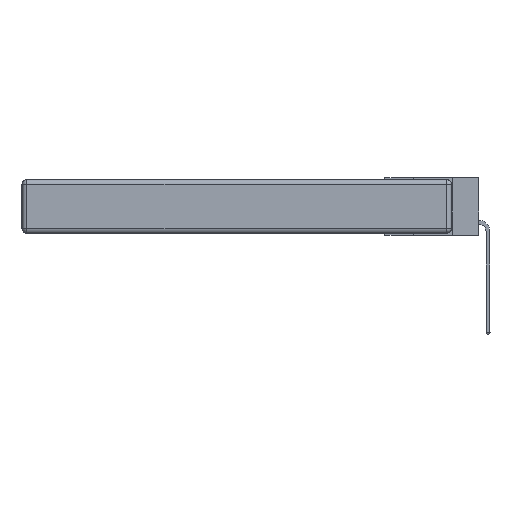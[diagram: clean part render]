
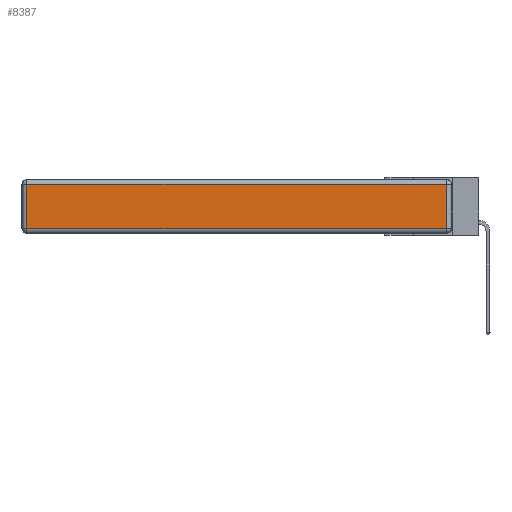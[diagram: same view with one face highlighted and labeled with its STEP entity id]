
A CAD part, left-side view. The second image highlights one B-rep face of the part: STEP entity #8387.
In plain terms, the highlighted planar face has unit normal (-1, 0, 0).
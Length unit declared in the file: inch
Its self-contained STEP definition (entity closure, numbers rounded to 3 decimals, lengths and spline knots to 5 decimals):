
#1116 = VECTOR ( 'NONE', #5650, 39.37008 ) ;
#1127 = VERTEX_POINT ( 'NONE', #4924 ) ;
#1510 = VECTOR ( 'NONE', #2442, 39.37008 ) ;
#1740 = ORIENTED_EDGE ( 'NONE', *, *, #8484, .T. ) ;
#2442 = DIRECTION ( 'NONE',  ( 0., 1., 0. ) ) ;
#3640 = EDGE_CURVE ( 'NONE', #12819, #5986, #6028, .T. ) ;
#4725 = DIRECTION ( 'NONE',  ( -1., 0., 0. ) ) ;
#4924 = CARTESIAN_POINT ( 'NONE',  ( 0., 2.72, -0.313 ) ) ;
#5626 = LINE ( 'NONE', #14146, #1116 ) ;
#5650 = DIRECTION ( 'NONE',  ( 0., 0., -1. ) ) ;
#5986 = VERTEX_POINT ( 'NONE', #17160 ) ;
#6028 = LINE ( 'NONE', #14596, #1510 ) ;
#6104 = VECTOR ( 'NONE', #10507, 39.37008 ) ;
#7439 = FACE_OUTER_BOUND ( 'NONE', #7593, .T. ) ;
#7593 = EDGE_LOOP ( 'NONE', ( #1740, #16730, #19042, #14198 ) ) ;
#8337 = CARTESIAN_POINT ( 'NONE',  ( 0., 0., -0.313 ) ) ;
#8387 = ADVANCED_FACE ( 'NONE', ( #7439 ), #18380, .T. ) ;
#8484 = EDGE_CURVE ( 'NONE', #1127, #9155, #21485, .T. ) ;
#9155 = VERTEX_POINT ( 'NONE', #18733 ) ;
#10507 = DIRECTION ( 'NONE',  ( 0., 0., 1. ) ) ;
#11314 = DIRECTION ( 'NONE',  ( 0., 0., 1. ) ) ;
#11346 = EDGE_CURVE ( 'NONE', #5986, #1127, #5626, .T. ) ;
#12456 = VECTOR ( 'NONE', #15246, 39.37008 ) ;
#12819 = VERTEX_POINT ( 'NONE', #14778 ) ;
#14146 = CARTESIAN_POINT ( 'NONE',  ( 0., 2.72, -0.343 ) ) ;
#14198 = ORIENTED_EDGE ( 'NONE', *, *, #11346, .T. ) ;
#14596 = CARTESIAN_POINT ( 'NONE',  ( 0., 2.75, -0.03 ) ) ;
#14778 = CARTESIAN_POINT ( 'NONE',  ( 0., 0.03, -0.03 ) ) ;
#15246 = DIRECTION ( 'NONE',  ( 0., -1., 0. ) ) ;
#16513 = CARTESIAN_POINT ( 'NONE',  ( 0., 0., -0.343 ) ) ;
#16722 = LINE ( 'NONE', #18870, #6104 ) ;
#16730 = ORIENTED_EDGE ( 'NONE', *, *, #17083, .T. ) ;
#17021 = AXIS2_PLACEMENT_3D ( 'NONE', #16513, #4725, #11314 ) ;
#17083 = EDGE_CURVE ( 'NONE', #9155, #12819, #16722, .T. ) ;
#17160 = CARTESIAN_POINT ( 'NONE',  ( 0., 2.72, -0.03 ) ) ;
#18380 = PLANE ( 'NONE',  #17021 ) ;
#18733 = CARTESIAN_POINT ( 'NONE',  ( 0., 0.03, -0.313 ) ) ;
#18870 = CARTESIAN_POINT ( 'NONE',  ( 0., 0.03, -0.343 ) ) ;
#19042 = ORIENTED_EDGE ( 'NONE', *, *, #3640, .T. ) ;
#21485 = LINE ( 'NONE', #8337, #12456 ) ;
